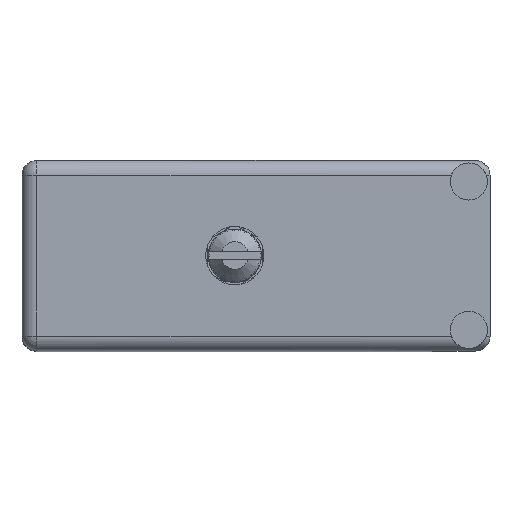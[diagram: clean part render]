
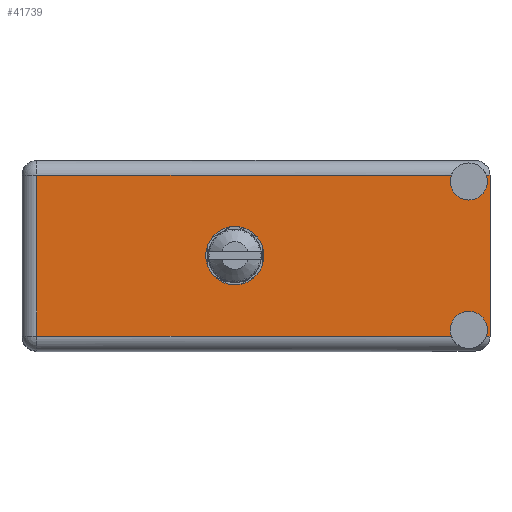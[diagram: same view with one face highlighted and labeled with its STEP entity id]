
A CAD part, top view. The second image highlights one B-rep face of the part: STEP entity #41739.
In plain terms, the highlighted face is planar.
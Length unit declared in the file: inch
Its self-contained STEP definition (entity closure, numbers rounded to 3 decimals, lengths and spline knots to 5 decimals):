
#1044 = VERTEX_POINT ( 'NONE', #33998 ) ;
#1300 = ORIENTED_EDGE ( 'NONE', *, *, #45742, .F. ) ;
#2927 = CARTESIAN_POINT ( 'NONE',  ( 1.204, 1.466, 0.3795 ) ) ;
#6411 = EDGE_CURVE ( 'NONE', #41859, #24230, #10234, .T. ) ;
#6761 = CARTESIAN_POINT ( 'NONE',  ( -1.004, 1.466, -0.3795 ) ) ;
#8867 = AXIS2_PLACEMENT_3D ( 'NONE', #48038, #23465, #80431 ) ;
#9691 = VECTOR ( 'NONE', #34392, 39.37008 ) ;
#10234 = LINE ( 'NONE', #6761, #62522 ) ;
#10903 = DIRECTION ( 'NONE',  ( 0., 0., 1. ) ) ;
#11034 = FACE_OUTER_BOUND ( 'NONE', #39149, .T. ) ;
#11310 = ORIENTED_EDGE ( 'NONE', *, *, #95136, .F. ) ;
#12838 = VECTOR ( 'NONE', #48729, 39.37008 ) ;
#15748 = DIRECTION ( 'NONE',  ( 0., 1., 0. ) ) ;
#16648 = CARTESIAN_POINT ( 'NONE',  ( 1.204, 1.466, 0.3795 ) ) ;
#18713 = FACE_BOUND ( 'NONE', #89679, .T. ) ;
#20903 = DIRECTION ( 'NONE',  ( 0., 0., 1. ) ) ;
#21632 = EDGE_CURVE ( 'NONE', #43124, #1044, #28300, .T. ) ;
#22356 = EDGE_CURVE ( 'NONE', #41859, #91046, #65281, .T. ) ;
#22468 = CIRCLE ( 'NONE', #29391, 0.0875 ) ;
#23043 = AXIS2_PLACEMENT_3D ( 'NONE', #58265, #50446, #83234 ) ;
#23465 = DIRECTION ( 'NONE',  ( 0., 1., 0. ) ) ;
#24230 = VERTEX_POINT ( 'NONE', #92625 ) ;
#24729 = ORIENTED_EDGE ( 'NONE', *, *, #21632, .F. ) ;
#25025 = VERTEX_POINT ( 'NONE', #65877 ) ;
#25372 = EDGE_CURVE ( 'NONE', #43799, #67074, #85473, .T. ) ;
#26393 = ORIENTED_EDGE ( 'NONE', *, *, #65333, .T. ) ;
#27969 = ORIENTED_EDGE ( 'NONE', *, *, #49866, .F. ) ;
#28177 = CARTESIAN_POINT ( 'NONE',  ( 1.18638, 1.466, 0.3795 ) ) ;
#28300 = LINE ( 'NONE', #50492, #47447 ) ;
#28594 = DIRECTION ( 'NONE',  ( 1., 0., 0. ) ) ;
#29094 = VERTEX_POINT ( 'NONE', #33077 ) ;
#29391 = AXIS2_PLACEMENT_3D ( 'NONE', #37572, #62527, #102734 ) ;
#31951 = CARTESIAN_POINT ( 'NONE',  ( -1.004, 1.466, -0.3795 ) ) ;
#32623 = AXIS2_PLACEMENT_3D ( 'NONE', #85937, #102578, #36008 ) ;
#33077 = CARTESIAN_POINT ( 'NONE',  ( 1.18638, 1.466, -0.3795 ) ) ;
#33543 = CARTESIAN_POINT ( 'NONE',  ( 1.104, 1.466, -0.2625 ) ) ;
#33998 = CARTESIAN_POINT ( 'NONE',  ( 1.204, 1.466, 0.3795 ) ) ;
#34392 = DIRECTION ( 'NONE',  ( 0., 0., 1. ) ) ;
#34747 = CARTESIAN_POINT ( 'NONE',  ( 1.104, 1.466, -0.35 ) ) ;
#35100 = CARTESIAN_POINT ( 'NONE',  ( -0.934, 1.466, -0.4495 ) ) ;
#36008 = DIRECTION ( 'NONE',  ( 0., 0., 1. ) ) ;
#36679 = ORIENTED_EDGE ( 'NONE', *, *, #6411, .T. ) ;
#37572 = CARTESIAN_POINT ( 'NONE',  ( 1.104, 1.466, 0.35 ) ) ;
#38105 = LINE ( 'NONE', #2927, #44469 ) ;
#39149 = EDGE_LOOP ( 'NONE', ( #42595, #87676, #80123, #80969, #24729, #26393, #11310, #88807, #36679, #98085 ) ) ;
#39316 = CARTESIAN_POINT ( 'NONE',  ( 1.204, 1.466, -0.3795 ) ) ;
#39571 = DIRECTION ( 'NONE',  ( 0., 0., 1. ) ) ;
#40271 = CARTESIAN_POINT ( 'NONE',  ( 0., 1.466, 0. ) ) ;
#41634 = CARTESIAN_POINT ( 'NONE',  ( 1.104, 1.466, 0.2625 ) ) ;
#41739 = ADVANCED_FACE ( 'NONE', ( #18713, #11034 ), #42924, .T. ) ;
#41859 = VERTEX_POINT ( 'NONE', #78235 ) ;
#42595 = ORIENTED_EDGE ( 'NONE', *, *, #25372, .T. ) ;
#42924 = PLANE ( 'NONE',  #23043 ) ;
#43124 = VERTEX_POINT ( 'NONE', #39316 ) ;
#43799 = VERTEX_POINT ( 'NONE', #63582 ) ;
#43851 = VECTOR ( 'NONE', #79731, 39.37008 ) ;
#44469 = VECTOR ( 'NONE', #28594, 39.37008 ) ;
#45742 = EDGE_CURVE ( 'NONE', #25025, #79036, #85577, .T. ) ;
#47302 = EDGE_CURVE ( 'NONE', #72326, #1044, #38105, .T. ) ;
#47447 = VECTOR ( 'NONE', #84673, 39.37008 ) ;
#47940 = LINE ( 'NONE', #35100, #9691 ) ;
#48038 = CARTESIAN_POINT ( 'NONE',  ( 1.104, 1.466, 0.35 ) ) ;
#48729 = DIRECTION ( 'NONE',  ( 1., 0., 0. ) ) ;
#49866 = EDGE_CURVE ( 'NONE', #79036, #25025, #95201, .T. ) ;
#50446 = DIRECTION ( 'NONE',  ( 0., 1., 0. ) ) ;
#50492 = CARTESIAN_POINT ( 'NONE',  ( 1.204, 1.466, 0.4495 ) ) ;
#51082 = EDGE_CURVE ( 'NONE', #72326, #86104, #22468, .T. ) ;
#56451 = EDGE_CURVE ( 'NONE', #24230, #43799, #47940, .T. ) ;
#57441 = AXIS2_PLACEMENT_3D ( 'NONE', #40271, #15748, #39571 ) ;
#57444 = EDGE_CURVE ( 'NONE', #86104, #67074, #83502, .T. ) ;
#58265 = CARTESIAN_POINT ( 'NONE',  ( -1.004, 1.466, -0.4495 ) ) ;
#62522 = VECTOR ( 'NONE', #78772, 39.37008 ) ;
#62527 = DIRECTION ( 'NONE',  ( 0., 1., 0. ) ) ;
#63582 = CARTESIAN_POINT ( 'NONE',  ( -0.934, 1.466, 0.3795 ) ) ;
#65281 = CIRCLE ( 'NONE', #83132, 0.0875 ) ;
#65333 = EDGE_CURVE ( 'NONE', #43124, #29094, #101163, .T. ) ;
#65877 = CARTESIAN_POINT ( 'NONE',  ( 0., 1.466, -0.1375 ) ) ;
#67074 = VERTEX_POINT ( 'NONE', #97191 ) ;
#68396 = AXIS2_PLACEMENT_3D ( 'NONE', #34747, #100934, #10903 ) ;
#68581 = DIRECTION ( 'NONE',  ( 0., 1., 0. ) ) ;
#72326 = VERTEX_POINT ( 'NONE', #28177 ) ;
#75411 = CARTESIAN_POINT ( 'NONE',  ( 0., 1.466, 0.1375 ) ) ;
#78235 = CARTESIAN_POINT ( 'NONE',  ( 1.02162, 1.466, -0.3795 ) ) ;
#78772 = DIRECTION ( 'NONE',  ( -1., 0., 0. ) ) ;
#79036 = VERTEX_POINT ( 'NONE', #75411 ) ;
#79731 = DIRECTION ( 'NONE',  ( -1., 0., 0. ) ) ;
#80123 = ORIENTED_EDGE ( 'NONE', *, *, #51082, .F. ) ;
#80431 = DIRECTION ( 'NONE',  ( 0., 0., 1. ) ) ;
#80969 = ORIENTED_EDGE ( 'NONE', *, *, #47302, .T. ) ;
#83132 = AXIS2_PLACEMENT_3D ( 'NONE', #86428, #68581, #20903 ) ;
#83234 = DIRECTION ( 'NONE',  ( -1., 0., 0. ) ) ;
#83502 = CIRCLE ( 'NONE', #8867, 0.0875 ) ;
#84673 = DIRECTION ( 'NONE',  ( 0., 0., 1. ) ) ;
#85473 = LINE ( 'NONE', #16648, #12838 ) ;
#85577 = CIRCLE ( 'NONE', #57441, 0.1375 ) ;
#85937 = CARTESIAN_POINT ( 'NONE',  ( 0., 1.466, 0. ) ) ;
#86104 = VERTEX_POINT ( 'NONE', #41634 ) ;
#86428 = CARTESIAN_POINT ( 'NONE',  ( 1.104, 1.466, -0.35 ) ) ;
#86437 = CIRCLE ( 'NONE', #68396, 0.0875 ) ;
#87676 = ORIENTED_EDGE ( 'NONE', *, *, #57444, .F. ) ;
#88807 = ORIENTED_EDGE ( 'NONE', *, *, #22356, .F. ) ;
#89679 = EDGE_LOOP ( 'NONE', ( #27969, #1300 ) ) ;
#91046 = VERTEX_POINT ( 'NONE', #33543 ) ;
#92625 = CARTESIAN_POINT ( 'NONE',  ( -0.934, 1.466, -0.3795 ) ) ;
#95136 = EDGE_CURVE ( 'NONE', #91046, #29094, #86437, .T. ) ;
#95201 = CIRCLE ( 'NONE', #32623, 0.1375 ) ;
#97191 = CARTESIAN_POINT ( 'NONE',  ( 1.02162, 1.466, 0.3795 ) ) ;
#98085 = ORIENTED_EDGE ( 'NONE', *, *, #56451, .T. ) ;
#100934 = DIRECTION ( 'NONE',  ( 0., 1., 0. ) ) ;
#101163 = LINE ( 'NONE', #31951, #43851 ) ;
#102578 = DIRECTION ( 'NONE',  ( 0., 1., 0. ) ) ;
#102734 = DIRECTION ( 'NONE',  ( 0., 0., 1. ) ) ;
